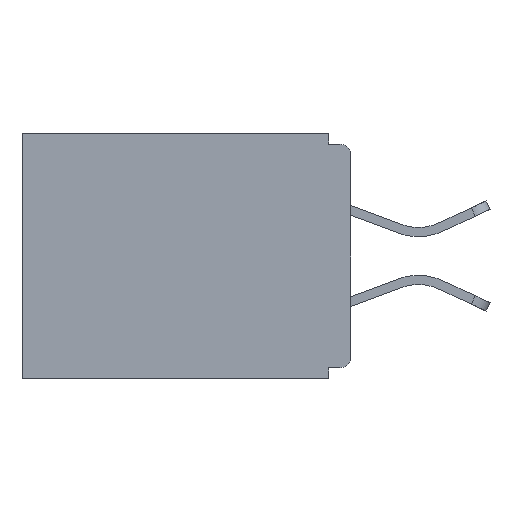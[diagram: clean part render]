
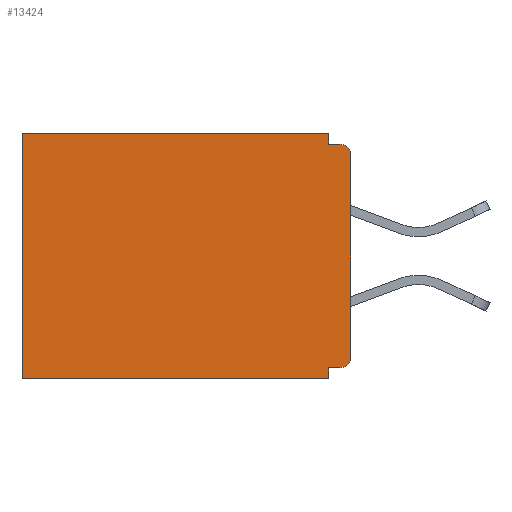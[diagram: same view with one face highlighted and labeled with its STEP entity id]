
A CAD part, left-side view. The second image highlights one B-rep face of the part: STEP entity #13424.
In plain terms, the highlighted planar face has unit normal (-1, 0, 0).
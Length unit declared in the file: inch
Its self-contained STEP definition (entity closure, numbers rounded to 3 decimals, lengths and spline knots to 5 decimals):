
#436 = CARTESIAN_POINT ( 'NONE',  ( 0.298, 0.031, -0.015 ) ) ;
#527 = CIRCLE ( 'NONE', #22993, 0.015 ) ;
#720 = DIRECTION ( 'NONE',  ( 0., 0., -1. ) ) ;
#760 = VECTOR ( 'NONE', #23745, 39.37008 ) ;
#863 = EDGE_CURVE ( 'NONE', #24058, #2431, #12703, .T. ) ;
#935 = ORIENTED_EDGE ( 'NONE', *, *, #4356, .F. ) ;
#968 = FACE_OUTER_BOUND ( 'NONE', #13996, .T. ) ;
#1904 = LINE ( 'NONE', #21697, #20744 ) ;
#1981 = CARTESIAN_POINT ( 'NONE',  ( 0.298, 0.031, 0. ) ) ;
#2431 = VERTEX_POINT ( 'NONE', #10324 ) ;
#2537 = ORIENTED_EDGE ( 'NONE', *, *, #21619, .F. ) ;
#2970 = VECTOR ( 'NONE', #7883, 39.37008 ) ;
#2997 = VERTEX_POINT ( 'NONE', #13954 ) ;
#3131 = EDGE_CURVE ( 'NONE', #2997, #4812, #4667, .T. ) ;
#3163 = CARTESIAN_POINT ( 'NONE',  ( 0.298, 0., -0.313 ) ) ;
#3615 = DIRECTION ( 'NONE',  ( 0., 1., 0. ) ) ;
#4181 = ORIENTED_EDGE ( 'NONE', *, *, #863, .T. ) ;
#4356 = EDGE_CURVE ( 'NONE', #4770, #24180, #22806, .T. ) ;
#4554 = PLANE ( 'NONE',  #8294 ) ;
#4584 = EDGE_CURVE ( 'NONE', #2997, #8467, #14909, .T. ) ;
#4667 = CIRCLE ( 'NONE', #10830, 0.015 ) ;
#4770 = VERTEX_POINT ( 'NONE', #436 ) ;
#4812 = VERTEX_POINT ( 'NONE', #3163 ) ;
#5230 = DIRECTION ( 'NONE',  ( 0., 0., -1. ) ) ;
#6469 = ORIENTED_EDGE ( 'NONE', *, *, #18047, .F. ) ;
#6615 = EDGE_CURVE ( 'NONE', #8001, #24180, #527, .T. ) ;
#7141 = ORIENTED_EDGE ( 'NONE', *, *, #16450, .F. ) ;
#7200 = VECTOR ( 'NONE', #11555, 39.37008 ) ;
#7883 = DIRECTION ( 'NONE',  ( 0., 0., -1. ) ) ;
#8001 = VERTEX_POINT ( 'NONE', #16522 ) ;
#8294 = AXIS2_PLACEMENT_3D ( 'NONE', #14935, #24467, #5230 ) ;
#8346 = CARTESIAN_POINT ( 'NONE',  ( 0.298, 0.46, 0. ) ) ;
#8467 = VERTEX_POINT ( 'NONE', #21494 ) ;
#8790 = CARTESIAN_POINT ( 'NONE',  ( 0.298, 0., -0.015 ) ) ;
#9241 = ORIENTED_EDGE ( 'NONE', *, *, #16567, .F. ) ;
#9377 = ORIENTED_EDGE ( 'NONE', *, *, #6615, .T. ) ;
#9675 = VECTOR ( 'NONE', #20363, 39.37008 ) ;
#10153 = DIRECTION ( 'NONE',  ( 0., 1., 0. ) ) ;
#10232 = CARTESIAN_POINT ( 'NONE',  ( 0.298, 0.015, -0.015 ) ) ;
#10324 = CARTESIAN_POINT ( 'NONE',  ( 0.298, 0.46, 0. ) ) ;
#10538 = DIRECTION ( 'NONE',  ( 0., 0., -1. ) ) ;
#10830 = AXIS2_PLACEMENT_3D ( 'NONE', #24019, #18320, #720 ) ;
#10888 = ORIENTED_EDGE ( 'NONE', *, *, #4584, .F. ) ;
#11555 = DIRECTION ( 'NONE',  ( 0., 0., -1. ) ) ;
#11586 = VERTEX_POINT ( 'NONE', #24580 ) ;
#11812 = CARTESIAN_POINT ( 'NONE',  ( 0.298, 0.031, -0.343 ) ) ;
#12051 = ORIENTED_EDGE ( 'NONE', *, *, #17280, .T. ) ;
#12594 = CARTESIAN_POINT ( 'NONE',  ( 0.298, 0.031, -0.343 ) ) ;
#12703 = LINE ( 'NONE', #16146, #12996 ) ;
#12843 = CARTESIAN_POINT ( 'NONE',  ( 0.298, 0.46, -0.343 ) ) ;
#12996 = VECTOR ( 'NONE', #17997, 39.37008 ) ;
#13073 = VECTOR ( 'NONE', #3615, 39.37008 ) ;
#13424 = ADVANCED_FACE ( 'NONE', ( #968 ), #4554, .F. ) ;
#13884 = LINE ( 'NONE', #8346, #760 ) ;
#13954 = CARTESIAN_POINT ( 'NONE',  ( 0.298, 0.015, -0.328 ) ) ;
#13996 = EDGE_LOOP ( 'NONE', ( #9377, #935, #6469, #4181, #12051, #2537, #9241, #10888, #17185, #7141 ) ) ;
#14289 = CARTESIAN_POINT ( 'NONE',  ( 0.298, 0.015, -0.03 ) ) ;
#14909 = LINE ( 'NONE', #15264, #13073 ) ;
#14935 = CARTESIAN_POINT ( 'NONE',  ( 0.298, 0., 0. ) ) ;
#15264 = CARTESIAN_POINT ( 'NONE',  ( 0.298, 0., -0.328 ) ) ;
#16146 = CARTESIAN_POINT ( 'NONE',  ( 0.298, 0., 0. ) ) ;
#16450 = EDGE_CURVE ( 'NONE', #8001, #4812, #23333, .T. ) ;
#16522 = CARTESIAN_POINT ( 'NONE',  ( 0.298, 0., -0.03 ) ) ;
#16567 = EDGE_CURVE ( 'NONE', #8467, #11586, #17266, .T. ) ;
#17185 = ORIENTED_EDGE ( 'NONE', *, *, #3131, .T. ) ;
#17266 = LINE ( 'NONE', #11812, #2970 ) ;
#17280 = EDGE_CURVE ( 'NONE', #2431, #23669, #13884, .T. ) ;
#17997 = DIRECTION ( 'NONE',  ( 0., 1., 0. ) ) ;
#18047 = EDGE_CURVE ( 'NONE', #24058, #4770, #20587, .T. ) ;
#18320 = DIRECTION ( 'NONE',  ( -1., 0., 0. ) ) ;
#20363 = DIRECTION ( 'NONE',  ( 0., 0., -1. ) ) ;
#20587 = LINE ( 'NONE', #12594, #9675 ) ;
#20744 = VECTOR ( 'NONE', #10153, 39.37008 ) ;
#21494 = CARTESIAN_POINT ( 'NONE',  ( 0.298, 0.031, -0.328 ) ) ;
#21619 = EDGE_CURVE ( 'NONE', #11586, #23669, #1904, .T. ) ;
#21697 = CARTESIAN_POINT ( 'NONE',  ( 0.298, 0., -0.343 ) ) ;
#22806 = LINE ( 'NONE', #8790, #23434 ) ;
#22993 = AXIS2_PLACEMENT_3D ( 'NONE', #14289, #24142, #10538 ) ;
#23253 = CARTESIAN_POINT ( 'NONE',  ( 0.298, 0., 0. ) ) ;
#23333 = LINE ( 'NONE', #23253, #7200 ) ;
#23434 = VECTOR ( 'NONE', #24375, 39.37008 ) ;
#23669 = VERTEX_POINT ( 'NONE', #12843 ) ;
#23745 = DIRECTION ( 'NONE',  ( 0., 0., -1. ) ) ;
#24019 = CARTESIAN_POINT ( 'NONE',  ( 0.298, 0.015, -0.313 ) ) ;
#24058 = VERTEX_POINT ( 'NONE', #1981 ) ;
#24142 = DIRECTION ( 'NONE',  ( -1., 0., 0. ) ) ;
#24180 = VERTEX_POINT ( 'NONE', #10232 ) ;
#24375 = DIRECTION ( 'NONE',  ( 0., -1., 0. ) ) ;
#24467 = DIRECTION ( 'NONE',  ( 1., 0., 0. ) ) ;
#24580 = CARTESIAN_POINT ( 'NONE',  ( 0.298, 0.031, -0.343 ) ) ;
